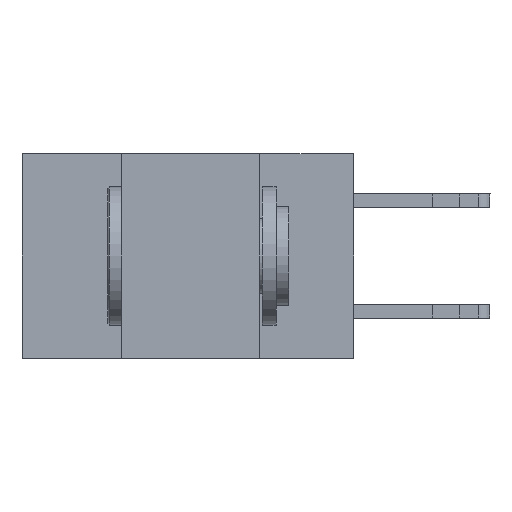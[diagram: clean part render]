
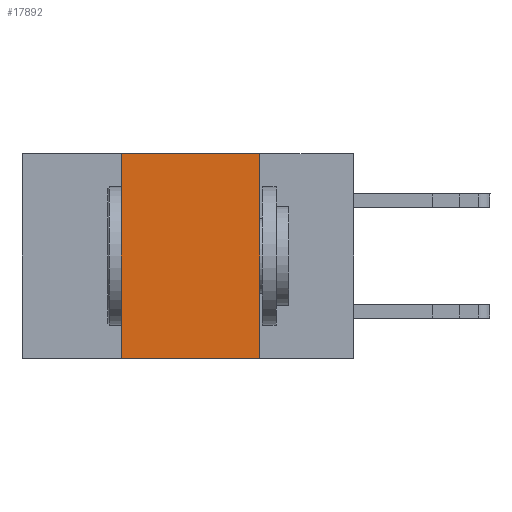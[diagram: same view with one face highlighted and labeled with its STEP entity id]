
A CAD part, left-side view. The second image highlights one B-rep face of the part: STEP entity #17892.
In plain terms, the highlighted planar face has unit normal (-1, 0, 0).
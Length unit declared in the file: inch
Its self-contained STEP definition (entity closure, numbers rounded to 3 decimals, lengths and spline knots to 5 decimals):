
#289 = VECTOR ( 'NONE', #2105, 39.37008 ) ;
#1758 = LINE ( 'NONE', #13335, #289 ) ;
#2105 = DIRECTION ( 'NONE',  ( 0., 0., 1. ) ) ;
#3560 = EDGE_CURVE ( 'NONE', #14526, #5462, #24481, .T. ) ;
#5312 = DIRECTION ( 'NONE',  ( 0., 0., -1. ) ) ;
#5462 = VERTEX_POINT ( 'NONE', #10899 ) ;
#5947 = FACE_OUTER_BOUND ( 'NONE', #24025, .T. ) ;
#6878 = ORIENTED_EDGE ( 'NONE', *, *, #22364, .T. ) ;
#6880 = CARTESIAN_POINT ( 'NONE',  ( 0., 0.42, -0.37 ) ) ;
#7134 = EDGE_CURVE ( 'NONE', #5462, #16563, #22740, .T. ) ;
#7328 = CARTESIAN_POINT ( 'NONE',  ( 0., 0.6, -0.37 ) ) ;
#7440 = CARTESIAN_POINT ( 'NONE',  ( 0., 0.6, 0. ) ) ;
#8024 = VECTOR ( 'NONE', #23476, 39.37008 ) ;
#8468 = AXIS2_PLACEMENT_3D ( 'NONE', #18902, #22669, #15416 ) ;
#9257 = ORIENTED_EDGE ( 'NONE', *, *, #7134, .F. ) ;
#9692 = ORIENTED_EDGE ( 'NONE', *, *, #3560, .F. ) ;
#9822 = CARTESIAN_POINT ( 'NONE',  ( 0., 0.17, -0.37 ) ) ;
#10899 = CARTESIAN_POINT ( 'NONE',  ( 0., 0.17, 0. ) ) ;
#11329 = PLANE ( 'NONE',  #8468 ) ;
#12098 = ORIENTED_EDGE ( 'NONE', *, *, #13148, .F. ) ;
#13148 = EDGE_CURVE ( 'NONE', #19840, #14526, #1758, .T. ) ;
#13335 = CARTESIAN_POINT ( 'NONE',  ( 0., 0.42, 0. ) ) ;
#14526 = VERTEX_POINT ( 'NONE', #20446 ) ;
#15056 = LINE ( 'NONE', #7328, #19755 ) ;
#15416 = DIRECTION ( 'NONE',  ( 0., 0., -1. ) ) ;
#16537 = VECTOR ( 'NONE', #5312, 39.37008 ) ;
#16563 = VERTEX_POINT ( 'NONE', #9822 ) ;
#17892 = ADVANCED_FACE ( 'NONE', ( #5947 ), #11329, .F. ) ;
#18902 = CARTESIAN_POINT ( 'NONE',  ( 0., 0.6, 0. ) ) ;
#19755 = VECTOR ( 'NONE', #22533, 39.37008 ) ;
#19840 = VERTEX_POINT ( 'NONE', #6880 ) ;
#20446 = CARTESIAN_POINT ( 'NONE',  ( 0., 0.42, 0. ) ) ;
#22364 = EDGE_CURVE ( 'NONE', #19840, #16563, #15056, .T. ) ;
#22533 = DIRECTION ( 'NONE',  ( 0., -1., 0. ) ) ;
#22669 = DIRECTION ( 'NONE',  ( 1., 0., 0. ) ) ;
#22740 = LINE ( 'NONE', #24349, #16537 ) ;
#23476 = DIRECTION ( 'NONE',  ( 0., -1., 0. ) ) ;
#24025 = EDGE_LOOP ( 'NONE', ( #9257, #9692, #12098, #6878 ) ) ;
#24349 = CARTESIAN_POINT ( 'NONE',  ( 0., 0.17, 0. ) ) ;
#24481 = LINE ( 'NONE', #7440, #8024 ) ;
